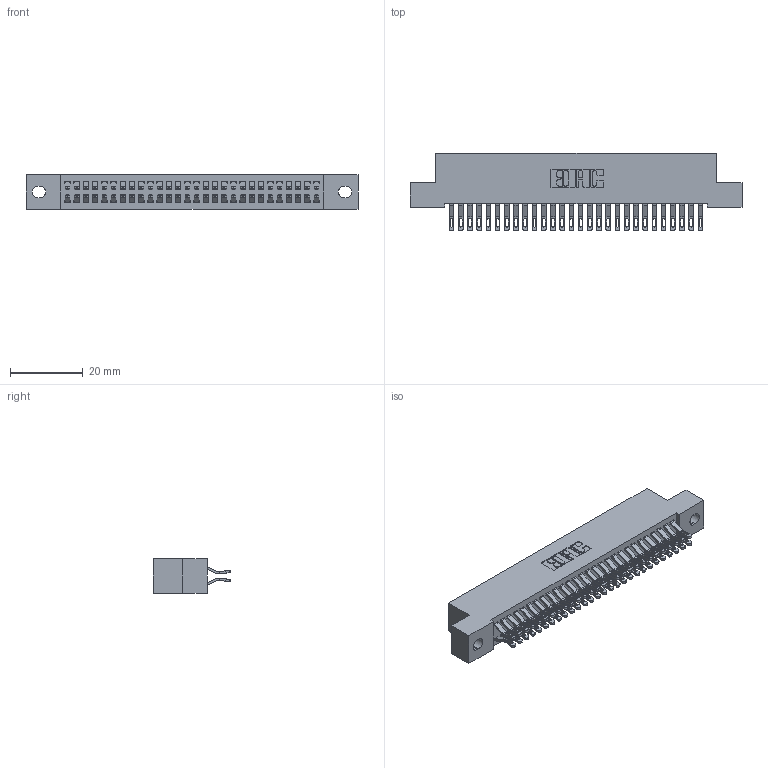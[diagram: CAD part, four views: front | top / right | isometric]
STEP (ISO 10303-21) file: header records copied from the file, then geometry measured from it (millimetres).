
FILE_DESCRIPTION (( 'STEP AP203' ), '1' );
FILE_NAME ('392-056-555-202.STEP', '2019-10-08T15:23:32', ( '' ), ( '' ), 'SwSTEP 2.0', 'SolidWorks 2016', '' );
FILE_SCHEMA (( 'CONFIG_CONTROL_DESIGN' ));
Length unit declared in the file: inch
Products named in the file (3): 342 Part_.128 Slot; 345-292-001_555 Tail; 392-056-555-202
Assembly tree (57 placements, depth 2):
  392-056-555-202
    342 Part_.128 Slot
    345-292-001_555 Tail  x56
Bounding box: 91.44 x 21.47 x 9.4 mm (x, y, z)
Volume: 8253.1 mm3; surface area: 13390.3 mm2
Topology: 57 solids, 57 shells, 3362 faces, 10559 edges, 7038 vertices
Faces by surface type: plane 1974, cylinder 1388
Entity records: 20153 total; most frequent: CARTESIAN_POINT 3392, ORIENTED_EDGE 3298, DIRECTION 2893, EDGE_CURVE 1649, VECTOR 1501, LINE 1501, VERTEX_POINT 1098, AXIS2_PLACEMENT_3D 696
